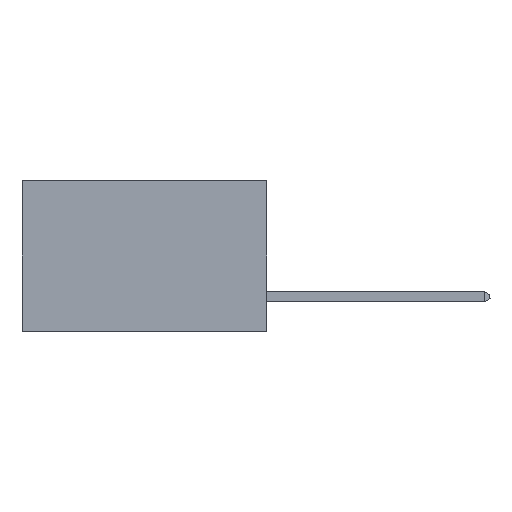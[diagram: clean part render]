
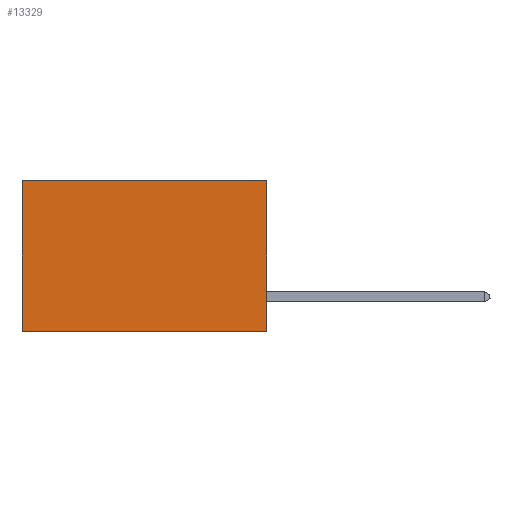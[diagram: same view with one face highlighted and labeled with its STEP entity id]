
A CAD part, left-side view. The second image highlights one B-rep face of the part: STEP entity #13329.
In plain terms, the highlighted planar face has unit normal (-1, 0, 0).
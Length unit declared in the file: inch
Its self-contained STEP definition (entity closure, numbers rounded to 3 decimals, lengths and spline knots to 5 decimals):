
#739 = EDGE_CURVE ( 'NONE', #5695, #4956, #12747, .T. ) ;
#795 = VECTOR ( 'NONE', #3493, 39.37008 ) ;
#1055 = DIRECTION ( 'NONE',  ( 1., 0., 0. ) ) ;
#2103 = CARTESIAN_POINT ( 'NONE',  ( 0.2875, 0.6, 0. ) ) ;
#2650 = DIRECTION ( 'NONE',  ( 0., 1., 0. ) ) ;
#3493 = DIRECTION ( 'NONE',  ( 0., 0., -1. ) ) ;
#3699 = ORIENTED_EDGE ( 'NONE', *, *, #10461, .T. ) ;
#4956 = VERTEX_POINT ( 'NONE', #17098 ) ;
#5695 = VERTEX_POINT ( 'NONE', #9201 ) ;
#5993 = ORIENTED_EDGE ( 'NONE', *, *, #7071, .T. ) ;
#6485 = PLANE ( 'NONE',  #9567 ) ;
#6923 = VECTOR ( 'NONE', #14783, 39.37008 ) ;
#7071 = EDGE_CURVE ( 'NONE', #13177, #10717, #13224, .T. ) ;
#7338 = LINE ( 'NONE', #13521, #6923 ) ;
#8198 = CARTESIAN_POINT ( 'NONE',  ( 0.2875, 0., 0. ) ) ;
#9072 = EDGE_LOOP ( 'NONE', ( #3699, #16900, #12925, #5993 ) ) ;
#9201 = CARTESIAN_POINT ( 'NONE',  ( 0.2875, 0., -0.37 ) ) ;
#9265 = VECTOR ( 'NONE', #2650, 39.37008 ) ;
#9567 = AXIS2_PLACEMENT_3D ( 'NONE', #13030, #1055, #10505 ) ;
#9782 = VECTOR ( 'NONE', #13430, 39.37008 ) ;
#10461 = EDGE_CURVE ( 'NONE', #10717, #4956, #11570, .T. ) ;
#10505 = DIRECTION ( 'NONE',  ( 0., 0., -1. ) ) ;
#10668 = FACE_OUTER_BOUND ( 'NONE', #9072, .T. ) ;
#10717 = VERTEX_POINT ( 'NONE', #14630 ) ;
#11570 = LINE ( 'NONE', #2103, #795 ) ;
#12697 = CARTESIAN_POINT ( 'NONE',  ( 0.2875, 0., 0. ) ) ;
#12747 = LINE ( 'NONE', #13170, #9265 ) ;
#12925 = ORIENTED_EDGE ( 'NONE', *, *, #15443, .F. ) ;
#13030 = CARTESIAN_POINT ( 'NONE',  ( 0.2875, 0., 0. ) ) ;
#13170 = CARTESIAN_POINT ( 'NONE',  ( 0.2875, 0., -0.37 ) ) ;
#13177 = VERTEX_POINT ( 'NONE', #12697 ) ;
#13224 = LINE ( 'NONE', #8198, #9782 ) ;
#13329 = ADVANCED_FACE ( 'NONE', ( #10668 ), #6485, .F. ) ;
#13430 = DIRECTION ( 'NONE',  ( 0., 1., 0. ) ) ;
#13521 = CARTESIAN_POINT ( 'NONE',  ( 0.2875, 0., 0. ) ) ;
#14630 = CARTESIAN_POINT ( 'NONE',  ( 0.2875, 0.6, 0. ) ) ;
#14783 = DIRECTION ( 'NONE',  ( 0., 0., -1. ) ) ;
#15443 = EDGE_CURVE ( 'NONE', #13177, #5695, #7338, .T. ) ;
#16900 = ORIENTED_EDGE ( 'NONE', *, *, #739, .F. ) ;
#17098 = CARTESIAN_POINT ( 'NONE',  ( 0.2875, 0.6, -0.37 ) ) ;
